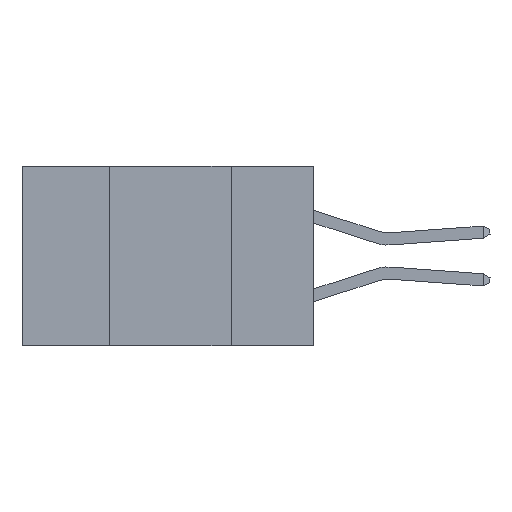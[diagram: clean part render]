
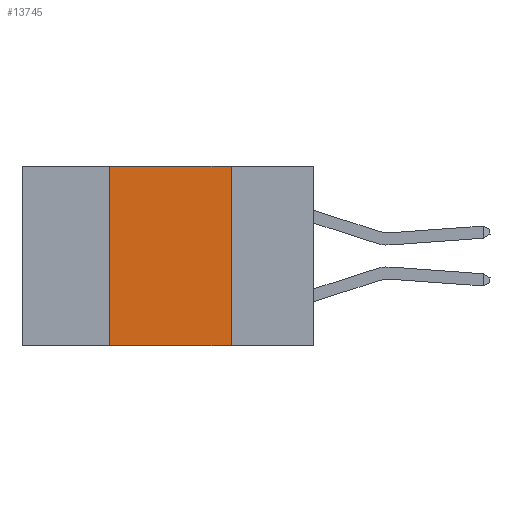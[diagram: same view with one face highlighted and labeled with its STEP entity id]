
A CAD part, left-side view. The second image highlights one B-rep face of the part: STEP entity #13745.
In plain terms, the highlighted planar face has unit normal (-1, 0, 0).
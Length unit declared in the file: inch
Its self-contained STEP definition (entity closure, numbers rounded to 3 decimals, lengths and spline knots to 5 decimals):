
#331 = VECTOR ( 'NONE', #3972, 39.37008 ) ;
#1319 = LINE ( 'NONE', #12270, #10139 ) ;
#1879 = EDGE_LOOP ( 'NONE', ( #18704, #10005, #5009, #3635 ) ) ;
#2159 = CARTESIAN_POINT ( 'NONE',  ( 0., 0.6, 0. ) ) ;
#2203 = EDGE_CURVE ( 'NONE', #11481, #3454, #1319, .T. ) ;
#2694 = LINE ( 'NONE', #21685, #23335 ) ;
#3454 = VERTEX_POINT ( 'NONE', #14031 ) ;
#3635 = ORIENTED_EDGE ( 'NONE', *, *, #2203, .T. ) ;
#3640 = DIRECTION ( 'NONE',  ( 0., 0., 1. ) ) ;
#3972 = DIRECTION ( 'NONE',  ( 0., -1., 0. ) ) ;
#4740 = VERTEX_POINT ( 'NONE', #13310 ) ;
#5009 = ORIENTED_EDGE ( 'NONE', *, *, #11866, .F. ) ;
#8175 = AXIS2_PLACEMENT_3D ( 'NONE', #10306, #17392, #15661 ) ;
#8620 = LINE ( 'NONE', #2159, #331 ) ;
#8690 = DIRECTION ( 'NONE',  ( 0., -1., 0. ) ) ;
#10005 = ORIENTED_EDGE ( 'NONE', *, *, #21789, .F. ) ;
#10139 = VECTOR ( 'NONE', #8690, 39.37008 ) ;
#10306 = CARTESIAN_POINT ( 'NONE',  ( 0., 0.6, 0. ) ) ;
#11481 = VERTEX_POINT ( 'NONE', #20318 ) ;
#11866 = EDGE_CURVE ( 'NONE', #11481, #4740, #2694, .T. ) ;
#12270 = CARTESIAN_POINT ( 'NONE',  ( 0., 0.6, -0.37 ) ) ;
#13109 = FACE_OUTER_BOUND ( 'NONE', #1879, .T. ) ;
#13178 = EDGE_CURVE ( 'NONE', #23012, #3454, #15643, .T. ) ;
#13310 = CARTESIAN_POINT ( 'NONE',  ( 0., 0.42, 0. ) ) ;
#13745 = ADVANCED_FACE ( 'NONE', ( #13109 ), #13877, .F. ) ;
#13877 = PLANE ( 'NONE',  #8175 ) ;
#14031 = CARTESIAN_POINT ( 'NONE',  ( 0., 0.17, -0.37 ) ) ;
#15643 = LINE ( 'NONE', #18277, #19296 ) ;
#15661 = DIRECTION ( 'NONE',  ( 0., 0., -1. ) ) ;
#17392 = DIRECTION ( 'NONE',  ( 1., 0., 0. ) ) ;
#18277 = CARTESIAN_POINT ( 'NONE',  ( 0., 0.17, 0. ) ) ;
#18704 = ORIENTED_EDGE ( 'NONE', *, *, #13178, .F. ) ;
#19296 = VECTOR ( 'NONE', #21625, 39.37008 ) ;
#20318 = CARTESIAN_POINT ( 'NONE',  ( 0., 0.42, -0.37 ) ) ;
#21625 = DIRECTION ( 'NONE',  ( 0., 0., -1. ) ) ;
#21685 = CARTESIAN_POINT ( 'NONE',  ( 0., 0.42, 0. ) ) ;
#21789 = EDGE_CURVE ( 'NONE', #4740, #23012, #8620, .T. ) ;
#23012 = VERTEX_POINT ( 'NONE', #23183 ) ;
#23183 = CARTESIAN_POINT ( 'NONE',  ( 0., 0.17, 0. ) ) ;
#23335 = VECTOR ( 'NONE', #3640, 39.37008 ) ;
